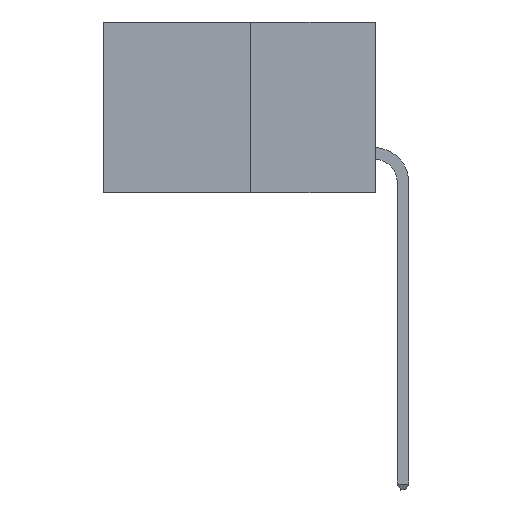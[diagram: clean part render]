
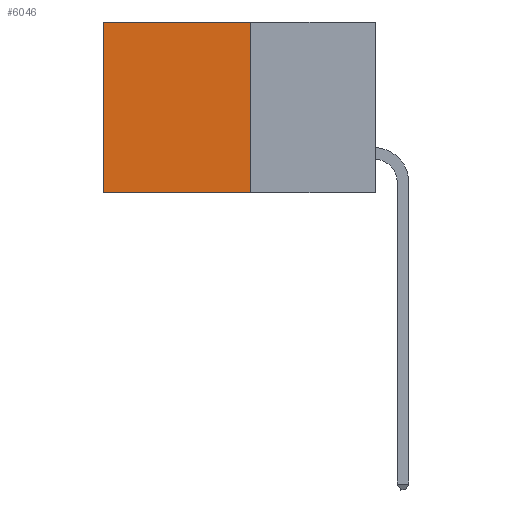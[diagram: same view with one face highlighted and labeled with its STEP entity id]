
A CAD part, left-side view. The second image highlights one B-rep face of the part: STEP entity #6046.
In plain terms, the highlighted planar face has unit normal (-1, 0, 0).
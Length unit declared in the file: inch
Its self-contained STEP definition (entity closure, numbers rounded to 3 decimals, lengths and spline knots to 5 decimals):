
#214 = VECTOR ( 'NONE', #974, 39.37008 ) ;
#974 = DIRECTION ( 'NONE',  ( 0., 0., -1. ) ) ;
#1456 = FACE_OUTER_BOUND ( 'NONE', #12235, .T. ) ;
#1820 = EDGE_CURVE ( 'NONE', #13344, #10664, #13361, .T. ) ;
#1968 = CARTESIAN_POINT ( 'NONE',  ( 0.277, 0.27, -0.37 ) ) ;
#3474 = LINE ( 'NONE', #6996, #214 ) ;
#4017 = CARTESIAN_POINT ( 'NONE',  ( 0.277, 0.27, 0. ) ) ;
#4098 = PLANE ( 'NONE',  #11536 ) ;
#4155 = DIRECTION ( 'NONE',  ( 1., 0., 0. ) ) ;
#4701 = CARTESIAN_POINT ( 'NONE',  ( 0.277, 0.27, -0.37 ) ) ;
#5581 = VERTEX_POINT ( 'NONE', #12874 ) ;
#6046 = ADVANCED_FACE ( 'NONE', ( #1456 ), #4098, .F. ) ;
#6706 = LINE ( 'NONE', #4017, #12765 ) ;
#6950 = VECTOR ( 'NONE', #15231, 39.37008 ) ;
#6996 = CARTESIAN_POINT ( 'NONE',  ( 0.277, 0.59, -0.37 ) ) ;
#7267 = ORIENTED_EDGE ( 'NONE', *, *, #1820, .F. ) ;
#10253 = EDGE_CURVE ( 'NONE', #13344, #5581, #6706, .T. ) ;
#10664 = VERTEX_POINT ( 'NONE', #4701 ) ;
#11197 = CARTESIAN_POINT ( 'NONE',  ( 0.277, 0.59, -0.37 ) ) ;
#11236 = DIRECTION ( 'NONE',  ( 0., 1., 0. ) ) ;
#11361 = CARTESIAN_POINT ( 'NONE',  ( 0.277, 0.27, -0.37 ) ) ;
#11512 = EDGE_CURVE ( 'NONE', #5581, #14924, #3474, .T. ) ;
#11536 = AXIS2_PLACEMENT_3D ( 'NONE', #11361, #4155, #12585 ) ;
#11579 = ORIENTED_EDGE ( 'NONE', *, *, #11512, .T. ) ;
#11681 = CARTESIAN_POINT ( 'NONE',  ( 0.277, 0.27, 0. ) ) ;
#12235 = EDGE_LOOP ( 'NONE', ( #11579, #12982, #7267, #14992 ) ) ;
#12585 = DIRECTION ( 'NONE',  ( 0., 0., -1. ) ) ;
#12765 = VECTOR ( 'NONE', #11236, 39.37008 ) ;
#12874 = CARTESIAN_POINT ( 'NONE',  ( 0.277, 0.59, 0. ) ) ;
#12982 = ORIENTED_EDGE ( 'NONE', *, *, #14574, .F. ) ;
#13027 = CARTESIAN_POINT ( 'NONE',  ( 0.277, 0.27, -0.37 ) ) ;
#13344 = VERTEX_POINT ( 'NONE', #11681 ) ;
#13361 = LINE ( 'NONE', #1968, #6950 ) ;
#14212 = DIRECTION ( 'NONE',  ( 0., 1., 0. ) ) ;
#14296 = VECTOR ( 'NONE', #14212, 39.37008 ) ;
#14574 = EDGE_CURVE ( 'NONE', #10664, #14924, #14664, .T. ) ;
#14664 = LINE ( 'NONE', #13027, #14296 ) ;
#14924 = VERTEX_POINT ( 'NONE', #11197 ) ;
#14992 = ORIENTED_EDGE ( 'NONE', *, *, #10253, .T. ) ;
#15231 = DIRECTION ( 'NONE',  ( 0., 0., -1. ) ) ;
